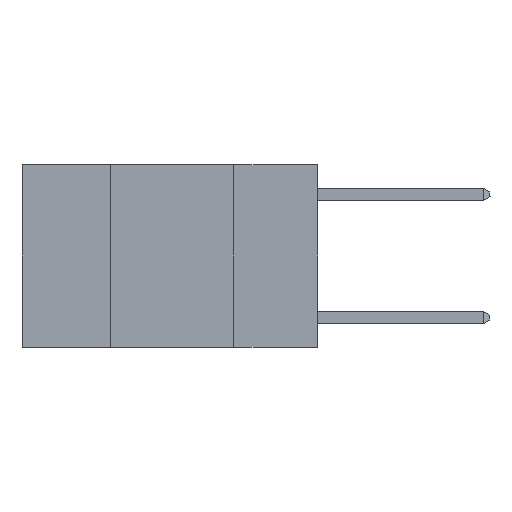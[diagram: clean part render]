
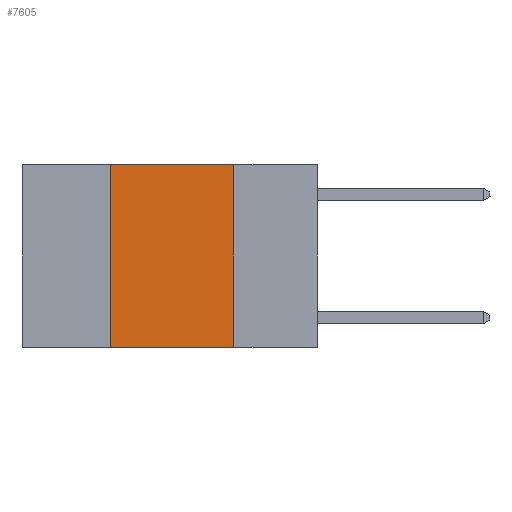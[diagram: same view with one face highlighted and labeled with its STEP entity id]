
A CAD part, left-side view. The second image highlights one B-rep face of the part: STEP entity #7605.
In plain terms, the highlighted planar face has unit normal (-1, 0, 0).
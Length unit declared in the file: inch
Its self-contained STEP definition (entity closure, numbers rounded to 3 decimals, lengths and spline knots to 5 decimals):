
#99 = LINE ( 'NONE', #3875, #9683 ) ;
#707 = EDGE_CURVE ( 'NONE', #8558, #4781, #9192, .T. ) ;
#716 = DIRECTION ( 'NONE',  ( 1., 0., 0. ) ) ;
#1085 = VERTEX_POINT ( 'NONE', #9470 ) ;
#1847 = LINE ( 'NONE', #9250, #4473 ) ;
#2030 = VECTOR ( 'NONE', #7115, 39.37008 ) ;
#2626 = PLANE ( 'NONE',  #5731 ) ;
#2823 = ORIENTED_EDGE ( 'NONE', *, *, #10953, .F. ) ;
#2900 = DIRECTION ( 'NONE',  ( 0., -1., 0. ) ) ;
#3343 = ORIENTED_EDGE ( 'NONE', *, *, #707, .T. ) ;
#3418 = VERTEX_POINT ( 'NONE', #3508 ) ;
#3508 = CARTESIAN_POINT ( 'NONE',  ( 0., 0.17, 0. ) ) ;
#3875 = CARTESIAN_POINT ( 'NONE',  ( 0., 0.42, 0. ) ) ;
#3960 = LINE ( 'NONE', #11680, #2030 ) ;
#4473 = VECTOR ( 'NONE', #6595, 39.37008 ) ;
#4616 = DIRECTION ( 'NONE',  ( 0., 0., 1. ) ) ;
#4781 = VERTEX_POINT ( 'NONE', #8217 ) ;
#5731 = AXIS2_PLACEMENT_3D ( 'NONE', #11796, #716, #8168 ) ;
#6059 = EDGE_LOOP ( 'NONE', ( #11832, #2823, #11285, #3343 ) ) ;
#6146 = CARTESIAN_POINT ( 'NONE',  ( 0., 0.42, -0.37 ) ) ;
#6595 = DIRECTION ( 'NONE',  ( 0., -1., 0. ) ) ;
#7115 = DIRECTION ( 'NONE',  ( 0., 0., -1. ) ) ;
#7520 = EDGE_CURVE ( 'NONE', #3418, #4781, #3960, .T. ) ;
#7605 = ADVANCED_FACE ( 'NONE', ( #8105 ), #2626, .F. ) ;
#8105 = FACE_OUTER_BOUND ( 'NONE', #6059, .T. ) ;
#8168 = DIRECTION ( 'NONE',  ( 0., 0., -1. ) ) ;
#8217 = CARTESIAN_POINT ( 'NONE',  ( 0., 0.17, -0.37 ) ) ;
#8558 = VERTEX_POINT ( 'NONE', #6146 ) ;
#9192 = LINE ( 'NONE', #11206, #9910 ) ;
#9250 = CARTESIAN_POINT ( 'NONE',  ( 0., 0.6, 0. ) ) ;
#9470 = CARTESIAN_POINT ( 'NONE',  ( 0., 0.42, 0. ) ) ;
#9683 = VECTOR ( 'NONE', #4616, 39.37008 ) ;
#9910 = VECTOR ( 'NONE', #2900, 39.37008 ) ;
#10082 = EDGE_CURVE ( 'NONE', #8558, #1085, #99, .T. ) ;
#10953 = EDGE_CURVE ( 'NONE', #1085, #3418, #1847, .T. ) ;
#11206 = CARTESIAN_POINT ( 'NONE',  ( 0., 0.6, -0.37 ) ) ;
#11285 = ORIENTED_EDGE ( 'NONE', *, *, #10082, .F. ) ;
#11680 = CARTESIAN_POINT ( 'NONE',  ( 0., 0.17, 0. ) ) ;
#11796 = CARTESIAN_POINT ( 'NONE',  ( 0., 0.6, 0. ) ) ;
#11832 = ORIENTED_EDGE ( 'NONE', *, *, #7520, .F. ) ;
